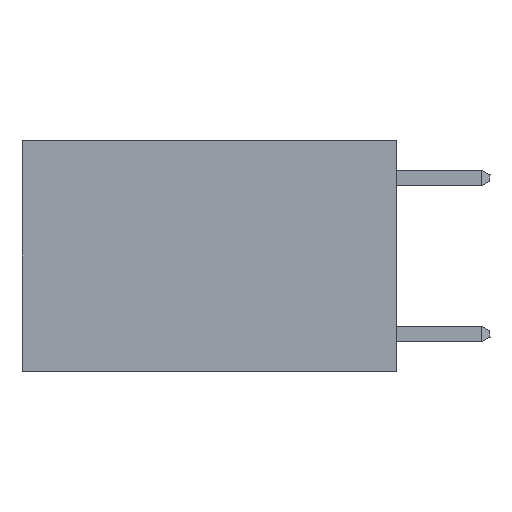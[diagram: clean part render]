
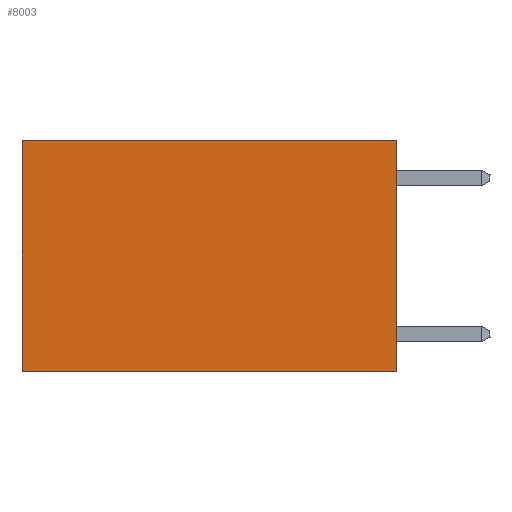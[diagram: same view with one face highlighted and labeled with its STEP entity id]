
A CAD part, left-side view. The second image highlights one B-rep face of the part: STEP entity #8003.
In plain terms, the highlighted planar face has unit normal (-1, 0, 0).
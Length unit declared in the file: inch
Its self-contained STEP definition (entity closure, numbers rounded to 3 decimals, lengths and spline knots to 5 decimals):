
#75 = EDGE_CURVE ( 'NONE', #6158, #20852, #20775, .T. ) ;
#581 = LINE ( 'NONE', #21647, #17015 ) ;
#1466 = DIRECTION ( 'NONE',  ( 1., 0., 0. ) ) ;
#1681 = VECTOR ( 'NONE', #8509, 39.37008 ) ;
#3090 = DIRECTION ( 'NONE',  ( 0., 1., 0. ) ) ;
#3167 = ORIENTED_EDGE ( 'NONE', *, *, #7427, .T. ) ;
#3795 = LINE ( 'NONE', #21235, #1681 ) ;
#3817 = EDGE_LOOP ( 'NONE', ( #3167, #7231, #18800, #19626 ) ) ;
#4510 = FACE_OUTER_BOUND ( 'NONE', #3817, .T. ) ;
#4578 = CARTESIAN_POINT ( 'NONE',  ( 0.2625, 0., -0.37 ) ) ;
#5026 = CARTESIAN_POINT ( 'NONE',  ( 0.2625, 0.6, -0.37 ) ) ;
#5709 = VERTEX_POINT ( 'NONE', #5026 ) ;
#6158 = VERTEX_POINT ( 'NONE', #18804 ) ;
#6815 = EDGE_CURVE ( 'NONE', #6158, #20448, #3795, .T. ) ;
#7231 = ORIENTED_EDGE ( 'NONE', *, *, #21472, .F. ) ;
#7427 = EDGE_CURVE ( 'NONE', #20852, #5709, #581, .T. ) ;
#7556 = AXIS2_PLACEMENT_3D ( 'NONE', #17077, #1466, #22089 ) ;
#8003 = ADVANCED_FACE ( 'NONE', ( #4510 ), #18321, .F. ) ;
#8509 = DIRECTION ( 'NONE',  ( 0., 0., -1. ) ) ;
#8986 = VECTOR ( 'NONE', #3090, 39.37008 ) ;
#10491 = DIRECTION ( 'NONE',  ( 0., 1., 0. ) ) ;
#12208 = CARTESIAN_POINT ( 'NONE',  ( 0.2625, 0., 0. ) ) ;
#12999 = DIRECTION ( 'NONE',  ( 0., 0., -1. ) ) ;
#14878 = CARTESIAN_POINT ( 'NONE',  ( 0.2625, 0.6, 0. ) ) ;
#17015 = VECTOR ( 'NONE', #12999, 39.37008 ) ;
#17077 = CARTESIAN_POINT ( 'NONE',  ( 0.2625, 0., 0. ) ) ;
#17243 = LINE ( 'NONE', #4578, #8986 ) ;
#17905 = CARTESIAN_POINT ( 'NONE',  ( 0.2625, 0., -0.37 ) ) ;
#18321 = PLANE ( 'NONE',  #7556 ) ;
#18800 = ORIENTED_EDGE ( 'NONE', *, *, #6815, .F. ) ;
#18804 = CARTESIAN_POINT ( 'NONE',  ( 0.2625, 0., 0. ) ) ;
#19626 = ORIENTED_EDGE ( 'NONE', *, *, #75, .T. ) ;
#20448 = VERTEX_POINT ( 'NONE', #17905 ) ;
#20775 = LINE ( 'NONE', #12208, #21204 ) ;
#20852 = VERTEX_POINT ( 'NONE', #14878 ) ;
#21204 = VECTOR ( 'NONE', #10491, 39.37008 ) ;
#21235 = CARTESIAN_POINT ( 'NONE',  ( 0.2625, 0., 0. ) ) ;
#21472 = EDGE_CURVE ( 'NONE', #20448, #5709, #17243, .T. ) ;
#21647 = CARTESIAN_POINT ( 'NONE',  ( 0.2625, 0.6, 0. ) ) ;
#22089 = DIRECTION ( 'NONE',  ( 0., 0., -1. ) ) ;
